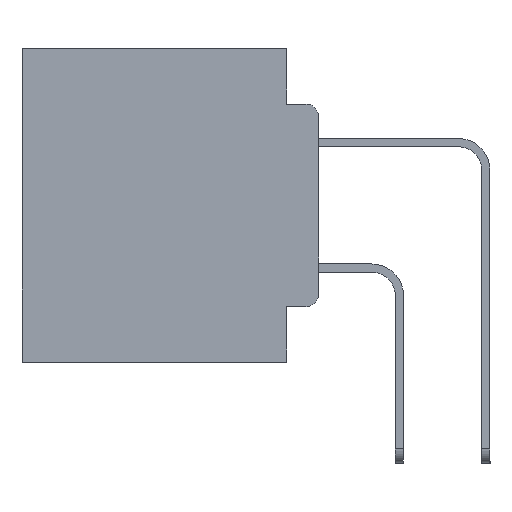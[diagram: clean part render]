
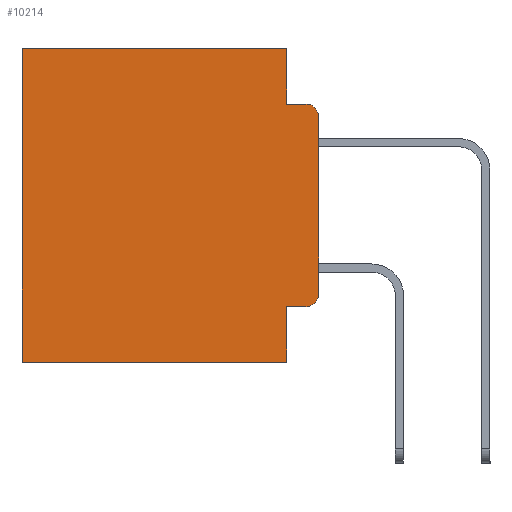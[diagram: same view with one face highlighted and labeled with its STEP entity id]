
A CAD part, left-side view. The second image highlights one B-rep face of the part: STEP entity #10214.
In plain terms, the highlighted planar face has unit normal (-1, 0, 0).
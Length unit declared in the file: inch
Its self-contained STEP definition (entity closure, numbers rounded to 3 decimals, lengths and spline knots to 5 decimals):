
#142 = CARTESIAN_POINT ( 'NONE',  ( 0.298, 0.051, 0. ) ) ;
#322 = VECTOR ( 'NONE', #22842, 39.37008 ) ;
#685 = LINE ( 'NONE', #24384, #4625 ) ;
#838 = VECTOR ( 'NONE', #25523, 39.37008 ) ;
#865 = CARTESIAN_POINT ( 'NONE',  ( 0.298, 0.02, -0.1085 ) ) ;
#1065 = EDGE_CURVE ( 'NONE', #14164, #22737, #10616, .T. ) ;
#1196 = VERTEX_POINT ( 'NONE', #9801 ) ;
#2000 = EDGE_CURVE ( 'NONE', #9307, #22737, #11266, .T. ) ;
#2318 = DIRECTION ( 'NONE',  ( 0., 0., -1. ) ) ;
#2846 = ORIENTED_EDGE ( 'NONE', *, *, #25387, .F. ) ;
#3007 = EDGE_CURVE ( 'NONE', #22822, #26206, #685, .T. ) ;
#3177 = EDGE_CURVE ( 'NONE', #26206, #17537, #19364, .T. ) ;
#3287 = DIRECTION ( 'NONE',  ( 0., 0., -1. ) ) ;
#3307 = DIRECTION ( 'NONE',  ( 0., 0., -1. ) ) ;
#3469 = CARTESIAN_POINT ( 'NONE',  ( 0.298, 0., -0.1085 ) ) ;
#4121 = DIRECTION ( 'NONE',  ( 0., 0., -1. ) ) ;
#4130 = EDGE_CURVE ( 'NONE', #9307, #1196, #7737, .T. ) ;
#4214 = DIRECTION ( 'NONE',  ( -1., 0., 0. ) ) ;
#4420 = CARTESIAN_POINT ( 'NONE',  ( 0.298, 0.051, -0.4115 ) ) ;
#4444 = DIRECTION ( 'NONE',  ( 0., 0., -1. ) ) ;
#4625 = VECTOR ( 'NONE', #27495, 39.37008 ) ;
#5602 = LINE ( 'NONE', #4420, #16693 ) ;
#6408 = EDGE_CURVE ( 'NONE', #9207, #10870, #6878, .T. ) ;
#6682 = DIRECTION ( 'NONE',  ( 0., -1., 0. ) ) ;
#6878 = LINE ( 'NONE', #142, #838 ) ;
#7410 = CARTESIAN_POINT ( 'NONE',  ( 0.298, 0.051, -0.4115 ) ) ;
#7737 = CIRCLE ( 'NONE', #17770, 0.02 ) ;
#8066 = CARTESIAN_POINT ( 'NONE',  ( 0.298, 0.02, -0.4115 ) ) ;
#8626 = CARTESIAN_POINT ( 'NONE',  ( 0.298, 0.051, -0.5 ) ) ;
#8971 = PLANE ( 'NONE',  #14827 ) ;
#9059 = CARTESIAN_POINT ( 'NONE',  ( 0.298, 0.473, -0.5 ) ) ;
#9207 = VERTEX_POINT ( 'NONE', #7410 ) ;
#9307 = VERTEX_POINT ( 'NONE', #3469 ) ;
#9775 = ORIENTED_EDGE ( 'NONE', *, *, #3007, .T. ) ;
#9801 = CARTESIAN_POINT ( 'NONE',  ( 0.298, 0.02, -0.0885 ) ) ;
#10040 = CARTESIAN_POINT ( 'NONE',  ( 0.298, 0., -0.3915 ) ) ;
#10195 = VECTOR ( 'NONE', #17709, 39.37008 ) ;
#10214 = ADVANCED_FACE ( 'NONE', ( #11568 ), #8971, .F. ) ;
#10492 = CARTESIAN_POINT ( 'NONE',  ( 0.298, 0., 0. ) ) ;
#10616 = CIRCLE ( 'NONE', #18795, 0.02 ) ;
#10870 = VERTEX_POINT ( 'NONE', #8626 ) ;
#11266 = LINE ( 'NONE', #10492, #21949 ) ;
#11289 = CARTESIAN_POINT ( 'NONE',  ( 0.298, 0., 0. ) ) ;
#11292 = CARTESIAN_POINT ( 'NONE',  ( 0.298, 0.02, -0.3915 ) ) ;
#11568 = FACE_OUTER_BOUND ( 'NONE', #15344, .T. ) ;
#12611 = EDGE_CURVE ( 'NONE', #22822, #14429, #19478, .T. ) ;
#13289 = ORIENTED_EDGE ( 'NONE', *, *, #3177, .T. ) ;
#13420 = CARTESIAN_POINT ( 'NONE',  ( 0.298, 0.051, -0.0885 ) ) ;
#13864 = VECTOR ( 'NONE', #3287, 39.37008 ) ;
#14164 = VERTEX_POINT ( 'NONE', #8066 ) ;
#14429 = VERTEX_POINT ( 'NONE', #13420 ) ;
#14492 = CARTESIAN_POINT ( 'NONE',  ( 0.298, 0., -0.5 ) ) ;
#14827 = AXIS2_PLACEMENT_3D ( 'NONE', #11289, #15705, #2318 ) ;
#15056 = CARTESIAN_POINT ( 'NONE',  ( 0.298, 0.473, 0. ) ) ;
#15100 = DIRECTION ( 'NONE',  ( 0., 0., -1. ) ) ;
#15344 = EDGE_LOOP ( 'NONE', ( #21547, #27375, #20502, #18784, #9775, #13289, #2846, #25543, #25066, #16771 ) ) ;
#15620 = CARTESIAN_POINT ( 'NONE',  ( 0.298, 0.051, -0.0885 ) ) ;
#15662 = EDGE_CURVE ( 'NONE', #9207, #14164, #5602, .T. ) ;
#15698 = EDGE_CURVE ( 'NONE', #14429, #1196, #27160, .T. ) ;
#15705 = DIRECTION ( 'NONE',  ( 1., 0., 0. ) ) ;
#16693 = VECTOR ( 'NONE', #6682, 39.37008 ) ;
#16771 = ORIENTED_EDGE ( 'NONE', *, *, #1065, .T. ) ;
#17537 = VERTEX_POINT ( 'NONE', #9059 ) ;
#17709 = DIRECTION ( 'NONE',  ( 0., -1., 0. ) ) ;
#17770 = AXIS2_PLACEMENT_3D ( 'NONE', #865, #4214, #4444 ) ;
#18023 = DIRECTION ( 'NONE',  ( -1., 0., 0. ) ) ;
#18784 = ORIENTED_EDGE ( 'NONE', *, *, #12611, .F. ) ;
#18795 = AXIS2_PLACEMENT_3D ( 'NONE', #11292, #18023, #4121 ) ;
#19364 = LINE ( 'NONE', #15056, #23608 ) ;
#19478 = LINE ( 'NONE', #24908, #13864 ) ;
#20502 = ORIENTED_EDGE ( 'NONE', *, *, #15698, .F. ) ;
#21109 = CARTESIAN_POINT ( 'NONE',  ( 0.298, 0.051, 0. ) ) ;
#21547 = ORIENTED_EDGE ( 'NONE', *, *, #2000, .F. ) ;
#21949 = VECTOR ( 'NONE', #3307, 39.37008 ) ;
#22737 = VERTEX_POINT ( 'NONE', #10040 ) ;
#22822 = VERTEX_POINT ( 'NONE', #21109 ) ;
#22842 = DIRECTION ( 'NONE',  ( 0., 1., 0. ) ) ;
#23435 = CARTESIAN_POINT ( 'NONE',  ( 0.298, 0.473, 0. ) ) ;
#23608 = VECTOR ( 'NONE', #15100, 39.37008 ) ;
#23613 = LINE ( 'NONE', #14492, #322 ) ;
#24384 = CARTESIAN_POINT ( 'NONE',  ( 0.298, 0., 0. ) ) ;
#24908 = CARTESIAN_POINT ( 'NONE',  ( 0.298, 0.051, 0. ) ) ;
#25066 = ORIENTED_EDGE ( 'NONE', *, *, #15662, .T. ) ;
#25387 = EDGE_CURVE ( 'NONE', #10870, #17537, #23613, .T. ) ;
#25523 = DIRECTION ( 'NONE',  ( 0., 0., -1. ) ) ;
#25543 = ORIENTED_EDGE ( 'NONE', *, *, #6408, .F. ) ;
#26206 = VERTEX_POINT ( 'NONE', #23435 ) ;
#27160 = LINE ( 'NONE', #15620, #10195 ) ;
#27375 = ORIENTED_EDGE ( 'NONE', *, *, #4130, .T. ) ;
#27495 = DIRECTION ( 'NONE',  ( 0., 1., 0. ) ) ;
